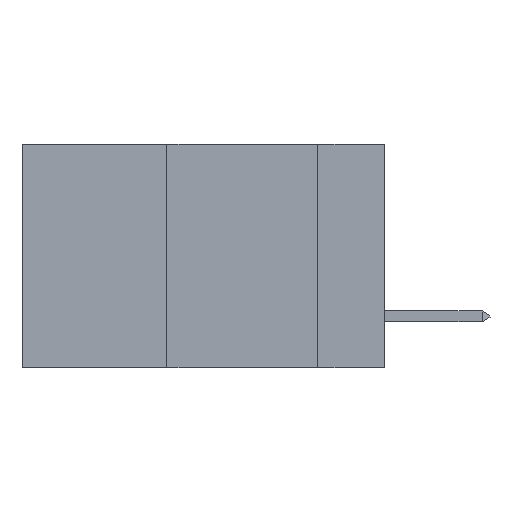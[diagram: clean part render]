
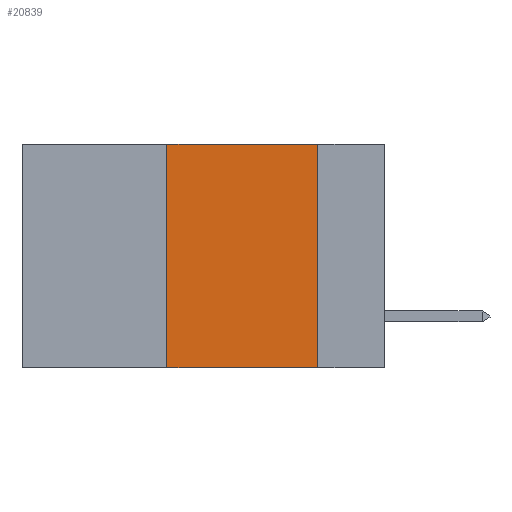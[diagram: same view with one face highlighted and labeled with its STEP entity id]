
A CAD part, left-side view. The second image highlights one B-rep face of the part: STEP entity #20839.
In plain terms, the highlighted planar face has unit normal (-1, 0, 0).
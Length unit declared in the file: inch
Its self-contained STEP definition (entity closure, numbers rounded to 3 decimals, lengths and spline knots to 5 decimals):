
#797 = ORIENTED_EDGE ( 'NONE', *, *, #2238, .F. ) ;
#2238 = EDGE_CURVE ( 'NONE', #8514, #17054, #21658, .T. ) ;
#2332 = CARTESIAN_POINT ( 'NONE',  ( 0., 0.36, 0. ) ) ;
#3084 = VECTOR ( 'NONE', #18254, 39.37008 ) ;
#3984 = VERTEX_POINT ( 'NONE', #2332 ) ;
#4006 = EDGE_CURVE ( 'NONE', #4277, #3984, #20518, .T. ) ;
#4277 = VERTEX_POINT ( 'NONE', #6622 ) ;
#4459 = DIRECTION ( 'NONE',  ( 0., -1., 0. ) ) ;
#5669 = VECTOR ( 'NONE', #10936, 39.37008 ) ;
#5881 = VECTOR ( 'NONE', #4459, 39.37008 ) ;
#6322 = ORIENTED_EDGE ( 'NONE', *, *, #21619, .F. ) ;
#6326 = CARTESIAN_POINT ( 'NONE',  ( 0., 0.6, 0. ) ) ;
#6622 = CARTESIAN_POINT ( 'NONE',  ( 0., 0.36, -0.37 ) ) ;
#7001 = CARTESIAN_POINT ( 'NONE',  ( 0., 0.11, 0. ) ) ;
#7461 = CARTESIAN_POINT ( 'NONE',  ( 0., 0.36, 0. ) ) ;
#7760 = PLANE ( 'NONE',  #18367 ) ;
#7822 = DIRECTION ( 'NONE',  ( 0., -1., 0. ) ) ;
#8514 = VERTEX_POINT ( 'NONE', #7001 ) ;
#9478 = DIRECTION ( 'NONE',  ( 0., 0., -1. ) ) ;
#9515 = CARTESIAN_POINT ( 'NONE',  ( 0., 0.6, -0.37 ) ) ;
#10039 = EDGE_CURVE ( 'NONE', #4277, #17054, #20473, .T. ) ;
#10607 = ORIENTED_EDGE ( 'NONE', *, *, #4006, .F. ) ;
#10936 = DIRECTION ( 'NONE',  ( 0., 0., 1. ) ) ;
#11187 = EDGE_LOOP ( 'NONE', ( #797, #6322, #10607, #12742 ) ) ;
#12742 = ORIENTED_EDGE ( 'NONE', *, *, #10039, .T. ) ;
#14665 = LINE ( 'NONE', #6326, #17865 ) ;
#15754 = FACE_OUTER_BOUND ( 'NONE', #11187, .T. ) ;
#17054 = VERTEX_POINT ( 'NONE', #18687 ) ;
#17865 = VECTOR ( 'NONE', #7822, 39.37008 ) ;
#18145 = CARTESIAN_POINT ( 'NONE',  ( 0., 0.6, 0. ) ) ;
#18254 = DIRECTION ( 'NONE',  ( 0., 0., -1. ) ) ;
#18367 = AXIS2_PLACEMENT_3D ( 'NONE', #18145, #19601, #9478 ) ;
#18687 = CARTESIAN_POINT ( 'NONE',  ( 0., 0.11, -0.37 ) ) ;
#19601 = DIRECTION ( 'NONE',  ( 1., 0., 0. ) ) ;
#20473 = LINE ( 'NONE', #9515, #5881 ) ;
#20518 = LINE ( 'NONE', #7461, #5669 ) ;
#20839 = ADVANCED_FACE ( 'NONE', ( #15754 ), #7760, .F. ) ;
#21619 = EDGE_CURVE ( 'NONE', #3984, #8514, #14665, .T. ) ;
#21658 = LINE ( 'NONE', #21692, #3084 ) ;
#21692 = CARTESIAN_POINT ( 'NONE',  ( 0., 0.11, 0. ) ) ;
